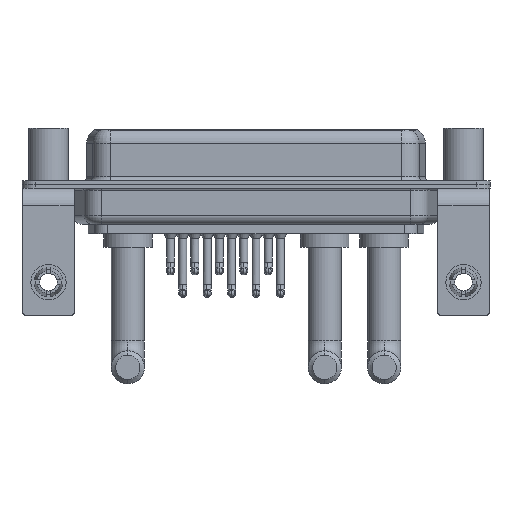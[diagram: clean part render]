
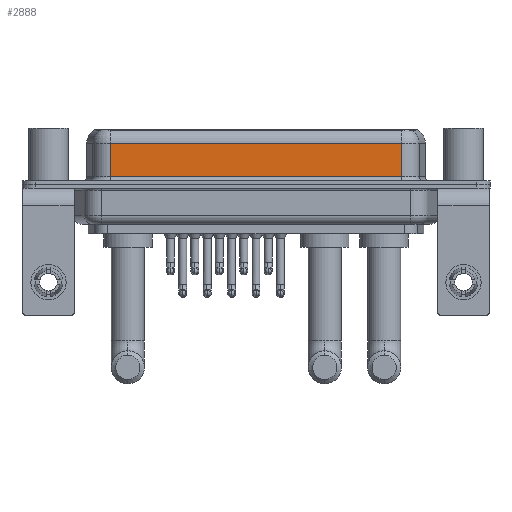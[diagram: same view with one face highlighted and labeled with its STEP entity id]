
A CAD part, front view. The second image highlights one B-rep face of the part: STEP entity #2888.
In plain terms, the highlighted planar face has unit normal (0, -1, 0).
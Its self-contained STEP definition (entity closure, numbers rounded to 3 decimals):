
#637 = EDGE_CURVE ( 'NONE', #15675, #20978, #9350, .T. ) ;
#1219 = PLANE ( 'NONE',  #14751 ) ;
#1534 = VECTOR ( 'NONE', #7417, 1000. ) ;
#1706 = EDGE_CURVE ( 'NONE', #10285, #2492, #11313, .T. ) ;
#2492 = VERTEX_POINT ( 'NONE', #21001 ) ;
#2846 = CARTESIAN_POINT ( 'NONE',  ( 40.037, -3.95, 0.9 ) ) ;
#2888 = ADVANCED_FACE ( 'NONE', ( #11594 ), #1219, .F. ) ;
#4020 = EDGE_CURVE ( 'NONE', #2492, #20978, #4278, .T. ) ;
#4278 = LINE ( 'NONE', #12747, #5480 ) ;
#4564 = EDGE_LOOP ( 'NONE', ( #12125, #14604, #13217, #12969 ) ) ;
#5455 = CARTESIAN_POINT ( 'NONE',  ( 40.037, -3.95, 6.4 ) ) ;
#5480 = VECTOR ( 'NONE', #19742, 1000. ) ;
#6966 = VECTOR ( 'NONE', #11542, 1000. ) ;
#7235 = CARTESIAN_POINT ( 'NONE',  ( 40.037, -3.95, 4.65 ) ) ;
#7417 = DIRECTION ( 'NONE',  ( 0., 0., -1. ) ) ;
#8434 = LINE ( 'NONE', #10256, #21063 ) ;
#9350 = LINE ( 'NONE', #5455, #1534 ) ;
#10256 = CARTESIAN_POINT ( 'NONE',  ( 40.037, -3.95, 4.65 ) ) ;
#10285 = VERTEX_POINT ( 'NONE', #21302 ) ;
#11313 = LINE ( 'NONE', #20480, #6966 ) ;
#11542 = DIRECTION ( 'NONE',  ( 0., 0., -1. ) ) ;
#11594 = FACE_OUTER_BOUND ( 'NONE', #4564, .T. ) ;
#12079 = DIRECTION ( 'NONE',  ( -1., 0., 0. ) ) ;
#12125 = ORIENTED_EDGE ( 'NONE', *, *, #637, .F. ) ;
#12679 = EDGE_CURVE ( 'NONE', #15675, #10285, #8434, .T. ) ;
#12747 = CARTESIAN_POINT ( 'NONE',  ( 40.037, -3.95, 0.9 ) ) ;
#12969 = ORIENTED_EDGE ( 'NONE', *, *, #4020, .T. ) ;
#13217 = ORIENTED_EDGE ( 'NONE', *, *, #1706, .T. ) ;
#14604 = ORIENTED_EDGE ( 'NONE', *, *, #12679, .T. ) ;
#14751 = AXIS2_PLACEMENT_3D ( 'NONE', #18694, #18580, #17105 ) ;
#15675 = VERTEX_POINT ( 'NONE', #7235 ) ;
#17105 = DIRECTION ( 'NONE',  ( 0., 0., 1. ) ) ;
#18580 = DIRECTION ( 'NONE',  ( 0., 1., 0. ) ) ;
#18694 = CARTESIAN_POINT ( 'NONE',  ( 40.037, -3.95, 6.4 ) ) ;
#19742 = DIRECTION ( 'NONE',  ( 1., 0., 0. ) ) ;
#20480 = CARTESIAN_POINT ( 'NONE',  ( 7.013, -3.95, 6.4 ) ) ;
#20978 = VERTEX_POINT ( 'NONE', #2846 ) ;
#21001 = CARTESIAN_POINT ( 'NONE',  ( 7.013, -3.95, 0.9 ) ) ;
#21063 = VECTOR ( 'NONE', #12079, 1000. ) ;
#21302 = CARTESIAN_POINT ( 'NONE',  ( 7.013, -3.95, 4.65 ) ) ;
